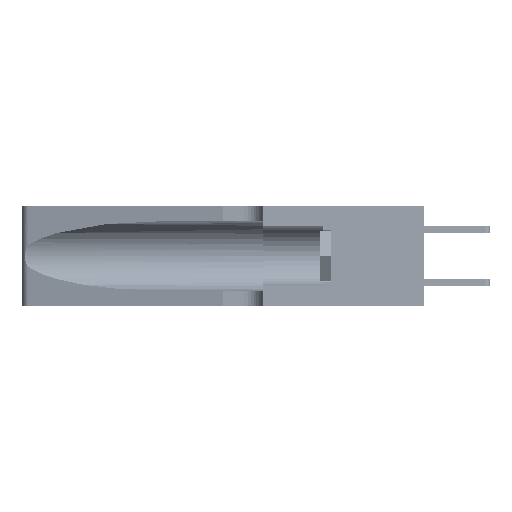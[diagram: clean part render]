
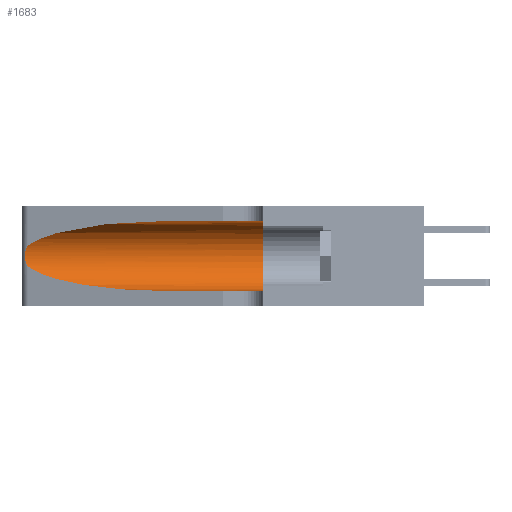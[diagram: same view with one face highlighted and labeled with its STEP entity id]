
A CAD part, left-side view. The second image highlights one B-rep face of the part: STEP entity #1683.
In plain terms, the highlighted cylindrical face has radius 3.308 mm (diameter 6.617 mm), a partial arc.
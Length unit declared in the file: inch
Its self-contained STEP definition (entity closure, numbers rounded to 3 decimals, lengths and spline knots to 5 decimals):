
#1683 = ADVANCED_FACE ( 'NONE', ( #33254 ), #38660, .F. ) ;
#1715 = CARTESIAN_POINT ( 'NONE',  ( 0.18966, 0.96281, 0.05475 ) ) ;
#3862 = ORIENTED_EDGE ( 'NONE', *, *, #33306, .F. ) ;
#4668 = ORIENTED_EDGE ( 'NONE', *, *, #35587, .T. ) ;
#5961 = CARTESIAN_POINT ( 'NONE',  ( 0.1305, 0.72297, 0.31525 ) ) ;
#6603 = CARTESIAN_POINT ( 'NONE',  ( 0.25639, 1.23184, 0.21858 ) ) ;
#6974 = EDGE_CURVE ( 'NONE', #12067, #17531, #45068, .T. ) ;
#7138 = AXIS2_PLACEMENT_3D ( 'NONE', #13594, #22206, #29282 ) ;
#9732 = EDGE_CURVE ( 'NONE', #13378, #41914, #30145, .T. ) ;
#10093 = VERTEX_POINT ( 'NONE', #31776 ) ;
#10303 = CARTESIAN_POINT ( 'NONE',  ( 0.1305, 0.35, 0.31525 ) ) ;
#11578 = CARTESIAN_POINT ( 'NONE',  ( 0.1305, 1.61858, 0.05475 ) ) ;
#12067 = VERTEX_POINT ( 'NONE', #22281 ) ;
#13378 = VERTEX_POINT ( 'NONE', #39750 ) ;
#13594 = CARTESIAN_POINT ( 'NONE',  ( 0.1305, 1.61858, 0.185 ) ) ;
#14660 = CARTESIAN_POINT ( 'NONE',  ( 0.1305, 0.72297, 0.05475 ) ) ;
#14921 = DIRECTION ( 'NONE',  ( 0., -1., 0. ) ) ;
#16394 = CARTESIAN_POINT ( 'NONE',  ( 0.1305, 0.72297, 0.05475 ) ) ;
#17270 = CARTESIAN_POINT ( 'NONE',  ( 0.2373, 1.15595, 0.28018 ) ) ;
#17531 = VERTEX_POINT ( 'NONE', #23888 ) ;
#17757 = CARTESIAN_POINT ( 'NONE',  ( 0.25487, 1.22718, 0.22369 ) ) ;
#21563 = CARTESIAN_POINT ( 'NONE',  ( 0.26018, 1.23835, 0.19895 ) ) ;
#21575 = DIRECTION ( 'NONE',  ( 0., 0., 1. ) ) ;
#22072 = DIRECTION ( 'NONE',  ( 0., 1., 0. ) ) ;
#22099 = ORIENTED_EDGE ( 'NONE', *, *, #9732, .F. ) ;
#22206 = DIRECTION ( 'NONE',  ( 0., -1., 0. ) ) ;
#22281 = CARTESIAN_POINT ( 'NONE',  ( 0.25487, 1.22718, 0.22369 ) ) ;
#23052 = EDGE_CURVE ( 'NONE', #41314, #10093, #25091, .T. ) ;
#23501 = CARTESIAN_POINT ( 'NONE',  ( 0.25487, 1.22718, 0.14631 ) ) ;
#23888 = CARTESIAN_POINT ( 'NONE',  ( 0.25487, 1.22718, 0.14631 ) ) ;
#24627 = CARTESIAN_POINT ( 'NONE',  ( 0.25555, 1.22994, 0.2215 ) ) ;
#24741 = ORIENTED_EDGE ( 'NONE', *, *, #6974, .T. ) ;
#25091 = LINE ( 'NONE', #11578, #38948 ) ;
#25602 = CIRCLE ( 'NONE', #46983, 0.13025 ) ;
#26500 =( BOUNDED_CURVE ( )  B_SPLINE_CURVE ( 3, ( #44078, #31937, #1715, #16394 ),
 .UNSPECIFIED., .F., .T. ) 
 B_SPLINE_CURVE_WITH_KNOTS ( ( 4, 4 ),
 ( 3.44316, 4.71239 ),
 .UNSPECIFIED. ) 
 CURVE ( )  GEOMETRIC_REPRESENTATION_ITEM ( )  RATIONAL_B_SPLINE_CURVE ( ( 1., 0.87, 0.87, 1. ) ) 
 REPRESENTATION_ITEM ( '' )  );
#29282 = DIRECTION ( 'NONE',  ( 0., 0., -1. ) ) ;
#30145 = LINE ( 'NONE', #49007, #32525 ) ;
#30835 = DIRECTION ( 'NONE',  ( 0., -1., 0. ) ) ;
#31758 =( BOUNDED_CURVE ( )  B_SPLINE_CURVE ( 3, ( #5961, #44462, #17270, #17757 ),
 .UNSPECIFIED., .F., .F. ) 
 B_SPLINE_CURVE_WITH_KNOTS ( ( 4, 4 ),
 ( 1.5708, 2.84003 ),
 .UNSPECIFIED. ) 
 CURVE ( )  GEOMETRIC_REPRESENTATION_ITEM ( )  RATIONAL_B_SPLINE_CURVE ( ( 1., 0.87, 0.87, 1. ) ) 
 REPRESENTATION_ITEM ( '' )  );
#31776 = CARTESIAN_POINT ( 'NONE',  ( 0.1305, 0.35, 0.05475 ) ) ;
#31937 = CARTESIAN_POINT ( 'NONE',  ( 0.2373, 1.15595, 0.08982 ) ) ;
#32525 = VECTOR ( 'NONE', #14921, 39.37008 ) ;
#32548 = CARTESIAN_POINT ( 'NONE',  ( 0.25487, 1.22718, 0.22369 ) ) ;
#33254 = FACE_OUTER_BOUND ( 'NONE', #44249, .T. ) ;
#33306 = EDGE_CURVE ( 'NONE', #41914, #10093, #25602, .T. ) ;
#35587 = EDGE_CURVE ( 'NONE', #17531, #41314, #26500, .T. ) ;
#35915 = CARTESIAN_POINT ( 'NONE',  ( 0.26017, 1.23833, 0.17102 ) ) ;
#36900 = CARTESIAN_POINT ( 'NONE',  ( 0.1305, 0.35, 0.185 ) ) ;
#38660 = CYLINDRICAL_SURFACE ( 'NONE', #7138, 0.13025 ) ;
#38948 = VECTOR ( 'NONE', #30835, 39.37008 ) ;
#39750 = CARTESIAN_POINT ( 'NONE',  ( 0.1305, 0.72297, 0.31525 ) ) ;
#41314 = VERTEX_POINT ( 'NONE', #14660 ) ;
#41502 = CARTESIAN_POINT ( 'NONE',  ( 0.25555, 1.22993, 0.14849 ) ) ;
#41914 = VERTEX_POINT ( 'NONE', #10303 ) ;
#42402 = CARTESIAN_POINT ( 'NONE',  ( 0.25856, 1.23593, 0.16098 ) ) ;
#42418 = CARTESIAN_POINT ( 'NONE',  ( 0.26075, 1.23896, 0.19203 ) ) ;
#43895 = CARTESIAN_POINT ( 'NONE',  ( 0.26075, 1.23896, 0.178 ) ) ;
#44078 = CARTESIAN_POINT ( 'NONE',  ( 0.25487, 1.22718, 0.14631 ) ) ;
#44249 = EDGE_LOOP ( 'NONE', ( #46440, #24741, #4668, #46339, #3862, #22099 ) ) ;
#44335 = CARTESIAN_POINT ( 'NONE',  ( 0.25854, 1.2359, 0.20912 ) ) ;
#44462 = CARTESIAN_POINT ( 'NONE',  ( 0.18966, 0.96281, 0.31525 ) ) ;
#45068 = B_SPLINE_CURVE_WITH_KNOTS ( 'NONE', 3,
 ( #32548, #24627, #6603, #48598, #44335, #21563, #42418, #43895, #35915, #42402, #49206, #48448, #41502, #23501 ),
 .UNSPECIFIED., .F., .F.,
 ( 4, 2, 2, 2, 2, 2, 4 ),
 ( 0., 0.00027, 0.00053, 0.00107, 0.0016, 0.00187, 0.00214 ),
 .UNSPECIFIED. ) ;
#45219 = EDGE_CURVE ( 'NONE', #13378, #12067, #31758, .T. ) ;
#46339 = ORIENTED_EDGE ( 'NONE', *, *, #23052, .T. ) ;
#46440 = ORIENTED_EDGE ( 'NONE', *, *, #45219, .T. ) ;
#46983 = AXIS2_PLACEMENT_3D ( 'NONE', #36900, #22072, #21575 ) ;
#48448 = CARTESIAN_POINT ( 'NONE',  ( 0.25639, 1.23186, 0.15144 ) ) ;
#48598 = CARTESIAN_POINT ( 'NONE',  ( 0.25787, 1.23484, 0.2124 ) ) ;
#49007 = CARTESIAN_POINT ( 'NONE',  ( 0.1305, 1.61858, 0.31525 ) ) ;
#49206 = CARTESIAN_POINT ( 'NONE',  ( 0.25789, 1.23486, 0.15765 ) ) ;
